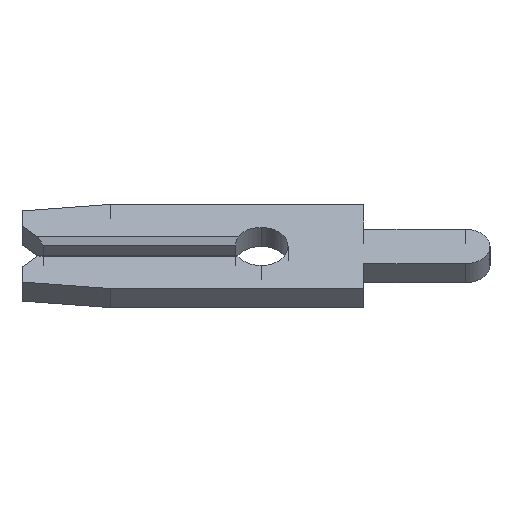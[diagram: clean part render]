
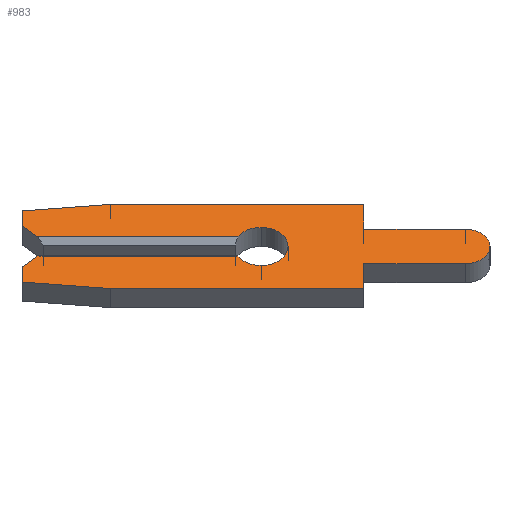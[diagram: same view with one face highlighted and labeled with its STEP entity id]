
A CAD part, left-side view. The second image highlights one B-rep face of the part: STEP entity #983.
In plain terms, the highlighted face is planar.
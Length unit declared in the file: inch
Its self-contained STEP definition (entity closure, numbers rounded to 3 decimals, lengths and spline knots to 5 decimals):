
#6 = LINE ( 'NONE', #748, #597 ) ;
#9 = CARTESIAN_POINT ( 'NONE',  ( -0.013, -0.099, -0.0235 ) ) ;
#16 = EDGE_CURVE ( 'NONE', #123, #1497, #747, .T. ) ;
#27 = DIRECTION ( 'NONE',  ( 0., 0., -1. ) ) ;
#31 = EDGE_CURVE ( 'NONE', #1625, #1644, #224, .T. ) ;
#38 = VECTOR ( 'NONE', #590, 39.37008 ) ;
#65 = CIRCLE ( 'NONE', #1215, 0.026 ) ;
#66 = DIRECTION ( 'NONE',  ( 0., 1., 0. ) ) ;
#77 = VERTEX_POINT ( 'NONE', #9 ) ;
#123 = VERTEX_POINT ( 'NONE', #1290 ) ;
#138 = DIRECTION ( 'NONE',  ( -1., 0., 0. ) ) ;
#152 = VERTEX_POINT ( 'NONE', #1632 ) ;
#185 = AXIS2_PLACEMENT_3D ( 'NONE', #1425, #138, #1428 ) ;
#207 = ORIENTED_EDGE ( 'NONE', *, *, #425, .F. ) ;
#218 = DIRECTION ( 'NONE',  ( -1., 0., 0. ) ) ;
#224 = LINE ( 'NONE', #1941, #1486 ) ;
#259 = ORIENTED_EDGE ( 'NONE', *, *, #918, .F. ) ;
#264 = ORIENTED_EDGE ( 'NONE', *, *, #16, .F. ) ;
#274 = LINE ( 'NONE', #866, #718 ) ;
#284 = ORIENTED_EDGE ( 'NONE', *, *, #1030, .F. ) ;
#309 = AXIS2_PLACEMENT_3D ( 'NONE', #1522, #218, #547 ) ;
#342 = VECTOR ( 'NONE', #66, 39.37008 ) ;
#348 = ORIENTED_EDGE ( 'NONE', *, *, #1579, .F. ) ;
#366 = DIRECTION ( 'NONE',  ( 0., 0., -1. ) ) ;
#370 = ORIENTED_EDGE ( 'NONE', *, *, #1935, .F. ) ;
#375 = CARTESIAN_POINT ( 'NONE',  ( -0.013, -0.099, 0.0575 ) ) ;
#386 = CIRCLE ( 'NONE', #1009, 0.0235 ) ;
#408 = DIRECTION ( 'NONE',  ( 0., 0., 1. ) ) ;
#415 = FACE_OUTER_BOUND ( 'NONE', #1845, .T. ) ;
#425 = EDGE_CURVE ( 'NONE', #152, #1698, #720, .T. ) ;
#426 = VERTEX_POINT ( 'NONE', #1511 ) ;
#433 = CARTESIAN_POINT ( 'NONE',  ( -0.013, 0.231, 0.028 ) ) ;
#450 = VERTEX_POINT ( 'NONE', #1335 ) ;
#462 = EDGE_CURVE ( 'NONE', #1725, #943, #1095, .T. ) ;
#466 = LINE ( 'NONE', #1378, #38 ) ;
#469 = VERTEX_POINT ( 'NONE', #1390 ) ;
#486 = CARTESIAN_POINT ( 'NONE',  ( -0.013, 0.231, 0.028 ) ) ;
#488 = EDGE_CURVE ( 'NONE', #426, #123, #466, .T. ) ;
#521 = VECTOR ( 'NONE', #1361, 39.37008 ) ;
#547 = DIRECTION ( 'NONE',  ( 0., 0., -1. ) ) ;
#548 = VECTOR ( 'NONE', #757, 39.37008 ) ;
#590 = DIRECTION ( 'NONE',  ( 0., 0., 1. ) ) ;
#597 = VECTOR ( 'NONE', #1756, 39.37008 ) ;
#598 = CARTESIAN_POINT ( 'NONE',  ( -0.013, 0.02252, 0.013 ) ) ;
#605 = EDGE_CURVE ( 'NONE', #1152, #1866, #1066, .T. ) ;
#645 = VECTOR ( 'NONE', #1228, 39.37008 ) ;
#674 = LINE ( 'NONE', #1028, #342 ) ;
#701 = ORIENTED_EDGE ( 'NONE', *, *, #1808, .F. ) ;
#711 = CARTESIAN_POINT ( 'NONE',  ( -0.013, -0.099, 0.0235 ) ) ;
#718 = VECTOR ( 'NONE', #2006, 39.37008 ) ;
#720 = CIRCLE ( 'NONE', #309, 0.026 ) ;
#730 = CARTESIAN_POINT ( 'NONE',  ( -0.013, 0.216, -0.013 ) ) ;
#735 = CARTESIAN_POINT ( 'NONE',  ( -0.013, 0.231, 0.04857 ) ) ;
#747 = LINE ( 'NONE', #1635, #1958 ) ;
#748 = CARTESIAN_POINT ( 'NONE',  ( -0.013, 0.231, 0.013 ) ) ;
#750 = ORIENTED_EDGE ( 'NONE', *, *, #783, .F. ) ;
#757 = DIRECTION ( 'NONE',  ( 0., -1., 0. ) ) ;
#764 = CARTESIAN_POINT ( 'NONE',  ( -0.013, 0.02252, -0.013 ) ) ;
#783 = EDGE_CURVE ( 'NONE', #1497, #1768, #1042, .T. ) ;
#798 = ORIENTED_EDGE ( 'NONE', *, *, #1800, .F. ) ;
#812 = LINE ( 'NONE', #486, #521 ) ;
#835 = AXIS2_PLACEMENT_3D ( 'NONE', #1128, #1645, #1492 ) ;
#839 = VECTOR ( 'NONE', #1710, 39.37008 ) ;
#866 = CARTESIAN_POINT ( 'NONE',  ( -0.013, 0.231, -0.04857 ) ) ;
#875 = ORIENTED_EDGE ( 'NONE', *, *, #1244, .F. ) ;
#907 = DIRECTION ( 'NONE',  ( 0., 0., -1. ) ) ;
#918 = EDGE_CURVE ( 'NONE', #1768, #1448, #65, .T. ) ;
#943 = VERTEX_POINT ( 'NONE', #1321 ) ;
#961 = ORIENTED_EDGE ( 'NONE', *, *, #605, .F. ) ;
#962 = DIRECTION ( 'NONE',  ( -1., 0., 0. ) ) ;
#983 = ADVANCED_FACE ( 'NONE', ( #415 ), #1316, .F. ) ;
#984 = LINE ( 'NONE', #1256, #548 ) ;
#1009 = AXIS2_PLACEMENT_3D ( 'NONE', #1040, #1376, #408 ) ;
#1028 = CARTESIAN_POINT ( 'NONE',  ( -0.013, -0.099, -0.0235 ) ) ;
#1030 = EDGE_CURVE ( 'NONE', #1644, #1152, #812, .T. ) ;
#1031 = ORIENTED_EDGE ( 'NONE', *, *, #1771, .T. ) ;
#1040 = CARTESIAN_POINT ( 'NONE',  ( -0.013, -0.1975, 0. ) ) ;
#1042 = LINE ( 'NONE', #1783, #1717 ) ;
#1061 = CARTESIAN_POINT ( 'NONE',  ( -0.013, 0.146, -0.0575 ) ) ;
#1064 = EDGE_CURVE ( 'NONE', #469, #1725, #1740, .T. ) ;
#1066 = LINE ( 'NONE', #735, #645 ) ;
#1094 = CARTESIAN_POINT ( 'NONE',  ( -0.013, -0.099, 0.0235 ) ) ;
#1095 = LINE ( 'NONE', #711, #839 ) ;
#1128 = CARTESIAN_POINT ( 'NONE',  ( -0.013, 0., 0. ) ) ;
#1141 = DIRECTION ( 'NONE',  ( 0., -0.707, 0.707 ) ) ;
#1142 = CARTESIAN_POINT ( 'NONE',  ( -0.013, 0., 0. ) ) ;
#1144 = VECTOR ( 'NONE', #907, 39.37008 ) ;
#1152 = VERTEX_POINT ( 'NONE', #2000 ) ;
#1215 = AXIS2_PLACEMENT_3D ( 'NONE', #1142, #962, #27 ) ;
#1228 = DIRECTION ( 'NONE',  ( 0., -0.995, 0.105 ) ) ;
#1230 = DIRECTION ( 'NONE',  ( 0., 1., 0. ) ) ;
#1244 = EDGE_CURVE ( 'NONE', #2043, #77, #674, .T. ) ;
#1256 = CARTESIAN_POINT ( 'NONE',  ( -0.013, 0.146, 0.0575 ) ) ;
#1275 = CARTESIAN_POINT ( 'NONE',  ( -0.013, -0.1975, -0.0235 ) ) ;
#1290 = CARTESIAN_POINT ( 'NONE',  ( -0.013, 0.231, -0.028 ) ) ;
#1301 = ORIENTED_EDGE ( 'NONE', *, *, #462, .F. ) ;
#1316 = PLANE ( 'NONE',  #835 ) ;
#1321 = CARTESIAN_POINT ( 'NONE',  ( -0.013, -0.1975, 0.0235 ) ) ;
#1335 = CARTESIAN_POINT ( 'NONE',  ( -0.013, -0.099, -0.0575 ) ) ;
#1361 = DIRECTION ( 'NONE',  ( 0., 0., 1. ) ) ;
#1376 = DIRECTION ( 'NONE',  ( 1., 0., 0. ) ) ;
#1378 = CARTESIAN_POINT ( 'NONE',  ( -0.013, 0.231, -0.028 ) ) ;
#1390 = CARTESIAN_POINT ( 'NONE',  ( -0.013, -0.099, 0.0575 ) ) ;
#1397 = CARTESIAN_POINT ( 'NONE',  ( -0.013, 0., -0.026 ) ) ;
#1410 = EDGE_CURVE ( 'NONE', #450, #1529, #1566, .T. ) ;
#1425 = CARTESIAN_POINT ( 'NONE',  ( -0.013, 0., 0. ) ) ;
#1428 = DIRECTION ( 'NONE',  ( 0., 0., -1. ) ) ;
#1435 = ORIENTED_EDGE ( 'NONE', *, *, #1064, .F. ) ;
#1448 = VERTEX_POINT ( 'NONE', #1397 ) ;
#1486 = VECTOR ( 'NONE', #1954, 39.37008 ) ;
#1492 = DIRECTION ( 'NONE',  ( 0., 0., -1. ) ) ;
#1497 = VERTEX_POINT ( 'NONE', #730 ) ;
#1511 = CARTESIAN_POINT ( 'NONE',  ( -0.013, 0.231, -0.04857 ) ) ;
#1514 = EDGE_CURVE ( 'NONE', #1529, #426, #274, .T. ) ;
#1516 = ORIENTED_EDGE ( 'NONE', *, *, #31, .F. ) ;
#1522 = CARTESIAN_POINT ( 'NONE',  ( -0.013, 0., 0. ) ) ;
#1529 = VERTEX_POINT ( 'NONE', #1853 ) ;
#1539 = CARTESIAN_POINT ( 'NONE',  ( -0.013, 0.216, 0.013 ) ) ;
#1543 = VECTOR ( 'NONE', #366, 39.37008 ) ;
#1566 = LINE ( 'NONE', #1061, #2053 ) ;
#1571 = ORIENTED_EDGE ( 'NONE', *, *, #488, .F. ) ;
#1579 = EDGE_CURVE ( 'NONE', #943, #2043, #386, .T. ) ;
#1583 = ORIENTED_EDGE ( 'NONE', *, *, #1514, .F. ) ;
#1593 = LINE ( 'NONE', #1745, #1144 ) ;
#1625 = VERTEX_POINT ( 'NONE', #1539 ) ;
#1632 = CARTESIAN_POINT ( 'NONE',  ( -0.013, 0., 0.026 ) ) ;
#1635 = CARTESIAN_POINT ( 'NONE',  ( -0.013, 0.2105, -0.0075 ) ) ;
#1636 = DIRECTION ( 'NONE',  ( 0., -1., 0. ) ) ;
#1644 = VERTEX_POINT ( 'NONE', #433 ) ;
#1645 = DIRECTION ( 'NONE',  ( 1., 0., 0. ) ) ;
#1698 = VERTEX_POINT ( 'NONE', #598 ) ;
#1710 = DIRECTION ( 'NONE',  ( 0., -1., 0. ) ) ;
#1717 = VECTOR ( 'NONE', #1636, 39.37008 ) ;
#1725 = VERTEX_POINT ( 'NONE', #1094 ) ;
#1736 = CARTESIAN_POINT ( 'NONE',  ( -0.013, 0.146, 0.0575 ) ) ;
#1740 = LINE ( 'NONE', #375, #1543 ) ;
#1745 = CARTESIAN_POINT ( 'NONE',  ( -0.013, -0.099, -0.0575 ) ) ;
#1756 = DIRECTION ( 'NONE',  ( 0., -1., 0. ) ) ;
#1760 = CIRCLE ( 'NONE', #185, 0.026 ) ;
#1768 = VERTEX_POINT ( 'NONE', #764 ) ;
#1771 = EDGE_CURVE ( 'NONE', #1625, #1698, #6, .T. ) ;
#1783 = CARTESIAN_POINT ( 'NONE',  ( -0.013, 0., -0.013 ) ) ;
#1792 = ORIENTED_EDGE ( 'NONE', *, *, #1410, .F. ) ;
#1800 = EDGE_CURVE ( 'NONE', #77, #450, #1593, .T. ) ;
#1808 = EDGE_CURVE ( 'NONE', #1866, #469, #984, .T. ) ;
#1845 = EDGE_LOOP ( 'NONE', ( #1031, #207, #370, #259, #750, #264, #1571, #1583, #1792, #798, #875, #348, #1301, #1435, #701, #961, #284, #1516 ) ) ;
#1853 = CARTESIAN_POINT ( 'NONE',  ( -0.013, 0.146, -0.0575 ) ) ;
#1866 = VERTEX_POINT ( 'NONE', #1736 ) ;
#1935 = EDGE_CURVE ( 'NONE', #1448, #152, #1760, .T. ) ;
#1941 = CARTESIAN_POINT ( 'NONE',  ( -0.013, 0.2105, 0.0075 ) ) ;
#1954 = DIRECTION ( 'NONE',  ( 0., 0.707, 0.707 ) ) ;
#1958 = VECTOR ( 'NONE', #1141, 39.37008 ) ;
#2000 = CARTESIAN_POINT ( 'NONE',  ( -0.013, 0.231, 0.04857 ) ) ;
#2006 = DIRECTION ( 'NONE',  ( 0., 0.995, 0.105 ) ) ;
#2043 = VERTEX_POINT ( 'NONE', #1275 ) ;
#2053 = VECTOR ( 'NONE', #1230, 39.37008 ) ;
